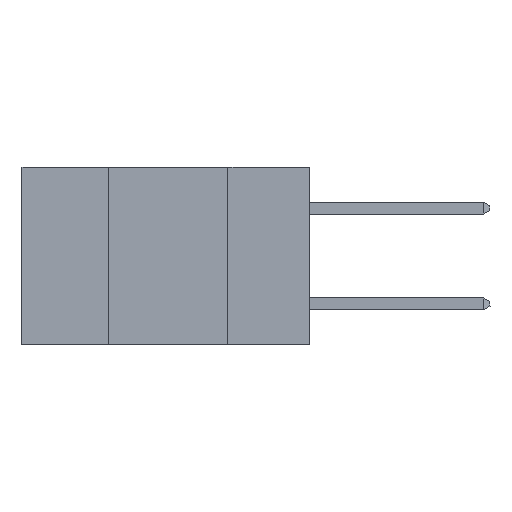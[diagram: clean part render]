
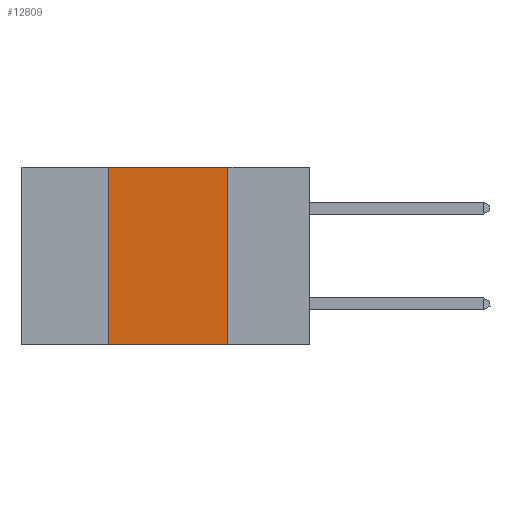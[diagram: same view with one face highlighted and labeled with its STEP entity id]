
A CAD part, left-side view. The second image highlights one B-rep face of the part: STEP entity #12809.
In plain terms, the highlighted planar face has unit normal (-1, 0, 0).
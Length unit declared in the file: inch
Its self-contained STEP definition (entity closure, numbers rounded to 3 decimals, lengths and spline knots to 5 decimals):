
#84 = CARTESIAN_POINT ( 'NONE',  ( 0., 0.42, -0.37 ) ) ;
#577 = CARTESIAN_POINT ( 'NONE',  ( 0., 0.6, 0. ) ) ;
#1586 = CARTESIAN_POINT ( 'NONE',  ( 0., 0.17, 0. ) ) ;
#1653 = VECTOR ( 'NONE', #6923, 39.37008 ) ;
#1687 = CARTESIAN_POINT ( 'NONE',  ( 0., 0.42, 0. ) ) ;
#1719 = EDGE_LOOP ( 'NONE', ( #6849, #19593, #5244, #5435 ) ) ;
#2856 = CARTESIAN_POINT ( 'NONE',  ( 0., 0.6, -0.37 ) ) ;
#3110 = LINE ( 'NONE', #1586, #7150 ) ;
#3921 = CARTESIAN_POINT ( 'NONE',  ( 0., 0.17, -0.37 ) ) ;
#5229 = EDGE_CURVE ( 'NONE', #16949, #20167, #18440, .T. ) ;
#5244 = ORIENTED_EDGE ( 'NONE', *, *, #18525, .F. ) ;
#5435 = ORIENTED_EDGE ( 'NONE', *, *, #21526, .T. ) ;
#6096 = VECTOR ( 'NONE', #12588, 39.37008 ) ;
#6120 = LINE ( 'NONE', #2856, #10623 ) ;
#6816 = DIRECTION ( 'NONE',  ( 0., 0., -1. ) ) ;
#6849 = ORIENTED_EDGE ( 'NONE', *, *, #6986, .F. ) ;
#6923 = DIRECTION ( 'NONE',  ( 0., 0., 1. ) ) ;
#6986 = EDGE_CURVE ( 'NONE', #20167, #8754, #3110, .T. ) ;
#7150 = VECTOR ( 'NONE', #6816, 39.37008 ) ;
#8754 = VERTEX_POINT ( 'NONE', #3921 ) ;
#8784 = CARTESIAN_POINT ( 'NONE',  ( 0., 0.6, 0. ) ) ;
#9401 = FACE_OUTER_BOUND ( 'NONE', #1719, .T. ) ;
#9527 = CARTESIAN_POINT ( 'NONE',  ( 0., 0.42, 0. ) ) ;
#10450 = DIRECTION ( 'NONE',  ( 0., 0., -1. ) ) ;
#10623 = VECTOR ( 'NONE', #14743, 39.37008 ) ;
#12588 = DIRECTION ( 'NONE',  ( 0., -1., 0. ) ) ;
#12809 = ADVANCED_FACE ( 'NONE', ( #9401 ), #13755, .F. ) ;
#13755 = PLANE ( 'NONE',  #18016 ) ;
#14743 = DIRECTION ( 'NONE',  ( 0., -1., 0. ) ) ;
#14807 = VERTEX_POINT ( 'NONE', #84 ) ;
#16179 = CARTESIAN_POINT ( 'NONE',  ( 0., 0.17, 0. ) ) ;
#16949 = VERTEX_POINT ( 'NONE', #9527 ) ;
#18016 = AXIS2_PLACEMENT_3D ( 'NONE', #8784, #20411, #10450 ) ;
#18440 = LINE ( 'NONE', #577, #6096 ) ;
#18525 = EDGE_CURVE ( 'NONE', #14807, #16949, #19104, .T. ) ;
#19104 = LINE ( 'NONE', #1687, #1653 ) ;
#19593 = ORIENTED_EDGE ( 'NONE', *, *, #5229, .F. ) ;
#20167 = VERTEX_POINT ( 'NONE', #16179 ) ;
#20411 = DIRECTION ( 'NONE',  ( 1., 0., 0. ) ) ;
#21526 = EDGE_CURVE ( 'NONE', #14807, #8754, #6120, .T. ) ;
